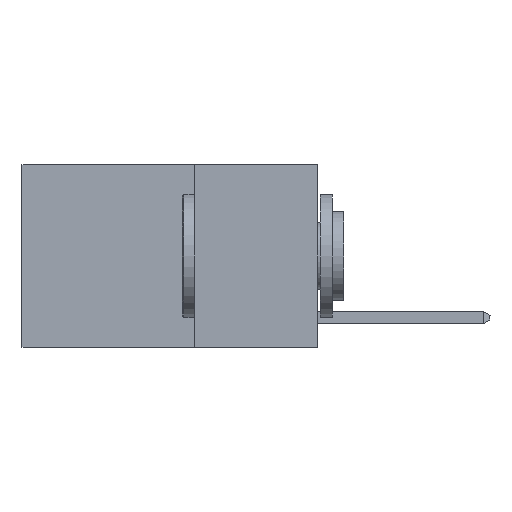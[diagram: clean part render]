
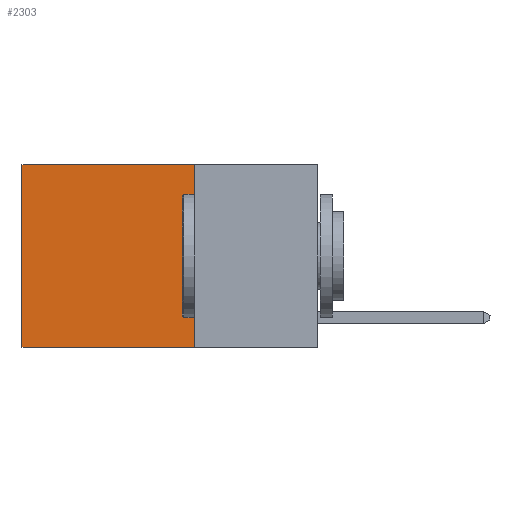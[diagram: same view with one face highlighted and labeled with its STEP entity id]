
A CAD part, left-side view. The second image highlights one B-rep face of the part: STEP entity #2303.
In plain terms, the highlighted planar face has unit normal (-1, 0, 0).
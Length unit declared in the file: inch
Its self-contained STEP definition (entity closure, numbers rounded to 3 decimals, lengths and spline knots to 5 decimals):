
#106 = ORIENTED_EDGE ( 'NONE', *, *, #5798, .T. ) ;
#360 = CARTESIAN_POINT ( 'NONE',  ( 0.2625, 0.6, 0. ) ) ;
#811 = CARTESIAN_POINT ( 'NONE',  ( 0.2625, 0.6, 0. ) ) ;
#1435 = VECTOR ( 'NONE', #5830, 39.37008 ) ;
#1739 = VECTOR ( 'NONE', #10626, 39.37008 ) ;
#1754 = CARTESIAN_POINT ( 'NONE',  ( 0.2625, 0.25, 0. ) ) ;
#1834 = VECTOR ( 'NONE', #6697, 39.37008 ) ;
#2196 = PLANE ( 'NONE',  #6690 ) ;
#2303 = ADVANCED_FACE ( 'NONE', ( #6486 ), #2196, .F. ) ;
#2399 = DIRECTION ( 'NONE',  ( 1., 0., 0. ) ) ;
#2504 = ORIENTED_EDGE ( 'NONE', *, *, #2734, .T. ) ;
#2514 = CARTESIAN_POINT ( 'NONE',  ( 0.2625, 0.25, -0.37 ) ) ;
#2539 = VERTEX_POINT ( 'NONE', #5177 ) ;
#2589 = ORIENTED_EDGE ( 'NONE', *, *, #6595, .F. ) ;
#2652 = LINE ( 'NONE', #1754, #1834 ) ;
#2734 = EDGE_CURVE ( 'NONE', #4887, #7660, #8982, .T. ) ;
#3096 = DIRECTION ( 'NONE',  ( 0., 0., -1. ) ) ;
#3366 = CARTESIAN_POINT ( 'NONE',  ( 0.2625, 0.6, -0.37 ) ) ;
#3921 = DIRECTION ( 'NONE',  ( 0., 0., -1. ) ) ;
#4887 = VERTEX_POINT ( 'NONE', #360 ) ;
#5177 = CARTESIAN_POINT ( 'NONE',  ( 0.2625, 0.25, 0. ) ) ;
#5789 = VERTEX_POINT ( 'NONE', #5826 ) ;
#5798 = EDGE_CURVE ( 'NONE', #2539, #4887, #2652, .T. ) ;
#5826 = CARTESIAN_POINT ( 'NONE',  ( 0.2625, 0.25, -0.37 ) ) ;
#5830 = DIRECTION ( 'NONE',  ( 0., 1., 0. ) ) ;
#6486 = FACE_OUTER_BOUND ( 'NONE', #10040, .T. ) ;
#6595 = EDGE_CURVE ( 'NONE', #2539, #5789, #8865, .T. ) ;
#6690 = AXIS2_PLACEMENT_3D ( 'NONE', #9778, #2399, #3921 ) ;
#6697 = DIRECTION ( 'NONE',  ( 0., 1., 0. ) ) ;
#7220 = CARTESIAN_POINT ( 'NONE',  ( 0.2625, 0.25, 0. ) ) ;
#7660 = VERTEX_POINT ( 'NONE', #3366 ) ;
#8865 = LINE ( 'NONE', #7220, #9081 ) ;
#8971 = EDGE_CURVE ( 'NONE', #5789, #7660, #9053, .T. ) ;
#8982 = LINE ( 'NONE', #811, #1739 ) ;
#9053 = LINE ( 'NONE', #2514, #1435 ) ;
#9081 = VECTOR ( 'NONE', #3096, 39.37008 ) ;
#9778 = CARTESIAN_POINT ( 'NONE',  ( 0.2625, 0.25, 0. ) ) ;
#9966 = ORIENTED_EDGE ( 'NONE', *, *, #8971, .F. ) ;
#10040 = EDGE_LOOP ( 'NONE', ( #2504, #9966, #2589, #106 ) ) ;
#10626 = DIRECTION ( 'NONE',  ( 0., 0., -1. ) ) ;
